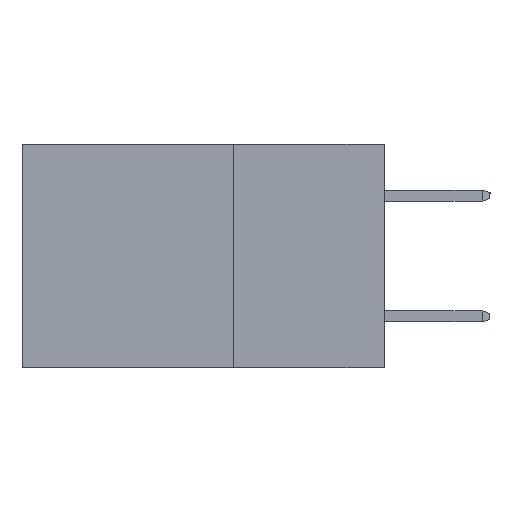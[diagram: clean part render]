
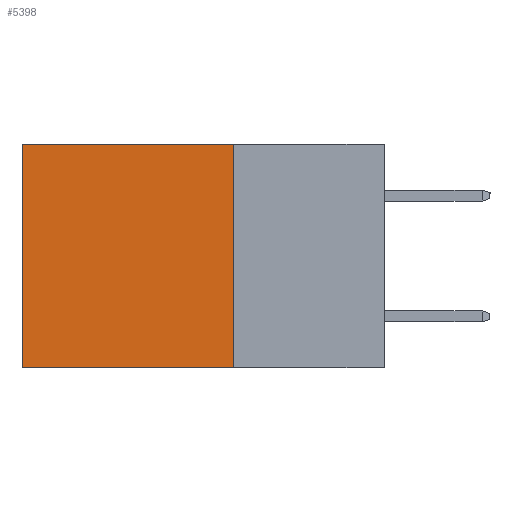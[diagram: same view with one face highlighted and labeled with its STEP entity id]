
A CAD part, left-side view. The second image highlights one B-rep face of the part: STEP entity #5398.
In plain terms, the highlighted planar face has unit normal (-1, 0, 0).
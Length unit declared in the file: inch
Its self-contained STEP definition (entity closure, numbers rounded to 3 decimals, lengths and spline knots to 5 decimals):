
#127 = VECTOR ( 'NONE', #10274, 39.37008 ) ;
#294 = VECTOR ( 'NONE', #3805, 39.37008 ) ;
#408 = DIRECTION ( 'NONE',  ( 1., 0., 0. ) ) ;
#529 = VECTOR ( 'NONE', #4617, 39.37008 ) ;
#852 = LINE ( 'NONE', #6614, #529 ) ;
#1574 = ORIENTED_EDGE ( 'NONE', *, *, #3773, .T. ) ;
#2390 = VERTEX_POINT ( 'NONE', #10787 ) ;
#2461 = CARTESIAN_POINT ( 'NONE',  ( 0.2615, 0.6, 0. ) ) ;
#3570 = VERTEX_POINT ( 'NONE', #2461 ) ;
#3773 = EDGE_CURVE ( 'NONE', #3570, #2390, #4220, .T. ) ;
#3805 = DIRECTION ( 'NONE',  ( 0., 0., -1. ) ) ;
#4220 = LINE ( 'NONE', #9138, #11273 ) ;
#4271 = VERTEX_POINT ( 'NONE', #11065 ) ;
#4617 = DIRECTION ( 'NONE',  ( 0., 1., 0. ) ) ;
#5398 = ADVANCED_FACE ( 'NONE', ( #6107 ), #9900, .F. ) ;
#6104 = EDGE_LOOP ( 'NONE', ( #1574, #10855, #11822, #6936 ) ) ;
#6107 = FACE_OUTER_BOUND ( 'NONE', #6104, .T. ) ;
#6614 = CARTESIAN_POINT ( 'NONE',  ( 0.2615, 0.25, -0.37 ) ) ;
#6936 = ORIENTED_EDGE ( 'NONE', *, *, #11614, .T. ) ;
#8047 = EDGE_CURVE ( 'NONE', #10221, #2390, #852, .T. ) ;
#8563 = LINE ( 'NONE', #11137, #294 ) ;
#8835 = EDGE_CURVE ( 'NONE', #4271, #10221, #8563, .T. ) ;
#8957 = CARTESIAN_POINT ( 'NONE',  ( 0.2615, 0.25, -0.37 ) ) ;
#9138 = CARTESIAN_POINT ( 'NONE',  ( 0.2615, 0.6, -0.37 ) ) ;
#9379 = DIRECTION ( 'NONE',  ( 0., 0., -1. ) ) ;
#9896 = CARTESIAN_POINT ( 'NONE',  ( 0.2615, 0.25, -0.37 ) ) ;
#9900 = PLANE ( 'NONE',  #11261 ) ;
#10221 = VERTEX_POINT ( 'NONE', #9896 ) ;
#10274 = DIRECTION ( 'NONE',  ( 0., 1., 0. ) ) ;
#10356 = LINE ( 'NONE', #11460, #127 ) ;
#10787 = CARTESIAN_POINT ( 'NONE',  ( 0.2615, 0.6, -0.37 ) ) ;
#10855 = ORIENTED_EDGE ( 'NONE', *, *, #8047, .F. ) ;
#11065 = CARTESIAN_POINT ( 'NONE',  ( 0.2615, 0.25, 0. ) ) ;
#11137 = CARTESIAN_POINT ( 'NONE',  ( 0.2615, 0.25, -0.37 ) ) ;
#11261 = AXIS2_PLACEMENT_3D ( 'NONE', #8957, #408, #9379 ) ;
#11273 = VECTOR ( 'NONE', #11835, 39.37008 ) ;
#11460 = CARTESIAN_POINT ( 'NONE',  ( 0.2615, 0.25, 0. ) ) ;
#11614 = EDGE_CURVE ( 'NONE', #4271, #3570, #10356, .T. ) ;
#11822 = ORIENTED_EDGE ( 'NONE', *, *, #8835, .F. ) ;
#11835 = DIRECTION ( 'NONE',  ( 0., 0., -1. ) ) ;
